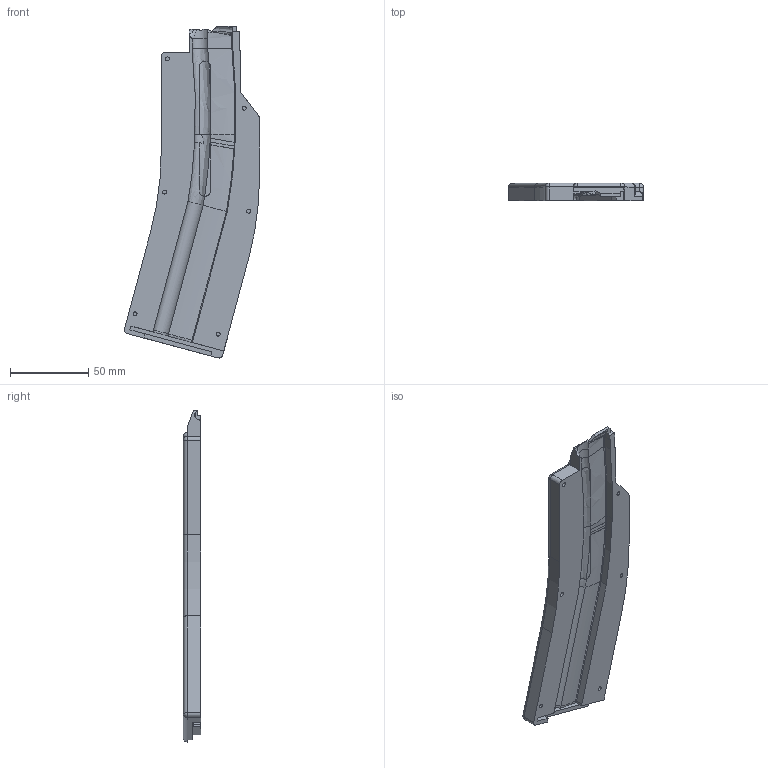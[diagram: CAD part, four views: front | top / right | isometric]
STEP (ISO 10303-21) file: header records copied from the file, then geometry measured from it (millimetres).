
FILE_DESCRIPTION(/* description */ (''),/* implementation_level */ '2;1');
FILE_NAME(/* name */ 'S&W 15-22 Right Mag 25r.step',/* time_stamp */ '2021-03-05T21:53:45-07:00',/* author */ (''),/* organization */ (''),/* preprocessor_version */ 'ST-DEVELOPER v18.1',/* originating_system */ 'Autodesk Translation Framework v9.10.0.1330',/* authorisation */ '');
FILE_SCHEMA (('AUTOMOTIVE_DESIGN { 1 0 10303 214 3 1 1 }'));
Length unit declared in the file: millimetre
Products named in the file (1): 22 Mag
Bounding box: 86.24 x 11.15 x 211.97 mm (x, y, z)
Volume: 107508.6 mm3; surface area: 32074.2 mm2
Topology: 1 solids, 1 shells, 167 faces, 414 edges, 253 vertices
Faces by surface type: plane 68, bspline 50, cylinder 41, sphere 6, torus 2
Full cylindrical faces by diameter (mm): 2.5 x6
Entity records: 6477 total; most frequent: CARTESIAN_POINT 2760, ORIENTED_EDGE 824, DIRECTION 673, EDGE_CURVE 412, VERTEX_POINT 253, AXIS2_PLACEMENT_3D 250, EDGE_LOOP 173, LINE 173
